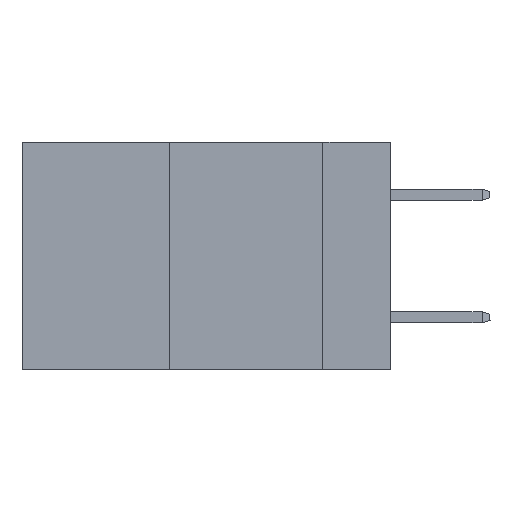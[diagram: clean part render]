
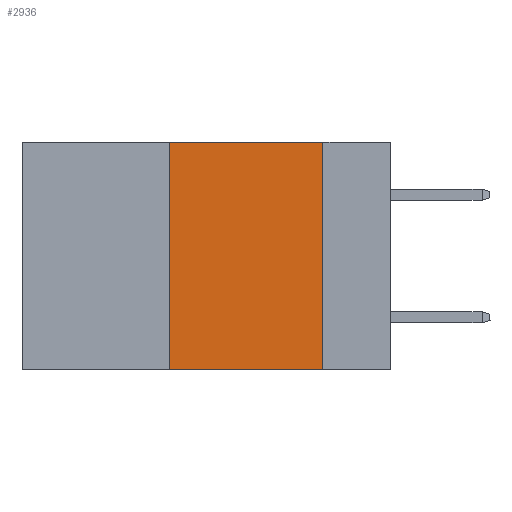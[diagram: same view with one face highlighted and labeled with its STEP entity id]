
A CAD part, left-side view. The second image highlights one B-rep face of the part: STEP entity #2936.
In plain terms, the highlighted planar face has unit normal (-1, 0, 0).
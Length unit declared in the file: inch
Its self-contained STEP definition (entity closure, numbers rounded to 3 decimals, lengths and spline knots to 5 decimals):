
#2936 = ADVANCED_FACE ( 'NONE', ( #44796 ), #31018, .F. ) ;
#3535 = ORIENTED_EDGE ( 'NONE', *, *, #41661, .F. ) ;
#3918 = CARTESIAN_POINT ( 'NONE',  ( 0., 0.36, -0.37 ) ) ;
#5176 = DIRECTION ( 'NONE',  ( 0., -1., 0. ) ) ;
#5412 = DIRECTION ( 'NONE',  ( 0., 0., 1. ) ) ;
#6112 = VECTOR ( 'NONE', #9706, 39.37008 ) ;
#6241 = EDGE_CURVE ( 'NONE', #44401, #22877, #20724, .T. ) ;
#6703 = EDGE_CURVE ( 'NONE', #9606, #19684, #37063, .T. ) ;
#7083 = DIRECTION ( 'NONE',  ( 0., 0., -1. ) ) ;
#8419 = CARTESIAN_POINT ( 'NONE',  ( 0., 0.36, 0. ) ) ;
#9606 = VERTEX_POINT ( 'NONE', #16468 ) ;
#9706 = DIRECTION ( 'NONE',  ( 0., 0., -1. ) ) ;
#11756 = VECTOR ( 'NONE', #5412, 39.37008 ) ;
#11927 = AXIS2_PLACEMENT_3D ( 'NONE', #21010, #17537, #7083 ) ;
#16468 = CARTESIAN_POINT ( 'NONE',  ( 0., 0.36, 0. ) ) ;
#17537 = DIRECTION ( 'NONE',  ( 1., 0., 0. ) ) ;
#19146 = VECTOR ( 'NONE', #21133, 39.37008 ) ;
#19684 = VERTEX_POINT ( 'NONE', #25856 ) ;
#20232 = ORIENTED_EDGE ( 'NONE', *, *, #6703, .F. ) ;
#20724 = LINE ( 'NONE', #43542, #36382 ) ;
#21010 = CARTESIAN_POINT ( 'NONE',  ( 0., 0.6, 0. ) ) ;
#21133 = DIRECTION ( 'NONE',  ( 0., -1., 0. ) ) ;
#22877 = VERTEX_POINT ( 'NONE', #42349 ) ;
#23512 = EDGE_LOOP ( 'NONE', ( #30982, #20232, #3535, #25848 ) ) ;
#25848 = ORIENTED_EDGE ( 'NONE', *, *, #6241, .T. ) ;
#25856 = CARTESIAN_POINT ( 'NONE',  ( 0., 0.11, 0. ) ) ;
#30982 = ORIENTED_EDGE ( 'NONE', *, *, #38725, .F. ) ;
#31018 = PLANE ( 'NONE',  #11927 ) ;
#31593 = CARTESIAN_POINT ( 'NONE',  ( 0., 0.6, 0. ) ) ;
#36189 = LINE ( 'NONE', #8419, #11756 ) ;
#36382 = VECTOR ( 'NONE', #5176, 39.37008 ) ;
#37063 = LINE ( 'NONE', #31593, #19146 ) ;
#38725 = EDGE_CURVE ( 'NONE', #19684, #22877, #44612, .T. ) ;
#41661 = EDGE_CURVE ( 'NONE', #44401, #9606, #36189, .T. ) ;
#42349 = CARTESIAN_POINT ( 'NONE',  ( 0., 0.11, -0.37 ) ) ;
#43542 = CARTESIAN_POINT ( 'NONE',  ( 0., 0.6, -0.37 ) ) ;
#44401 = VERTEX_POINT ( 'NONE', #3918 ) ;
#44419 = CARTESIAN_POINT ( 'NONE',  ( 0., 0.11, 0. ) ) ;
#44612 = LINE ( 'NONE', #44419, #6112 ) ;
#44796 = FACE_OUTER_BOUND ( 'NONE', #23512, .T. ) ;
